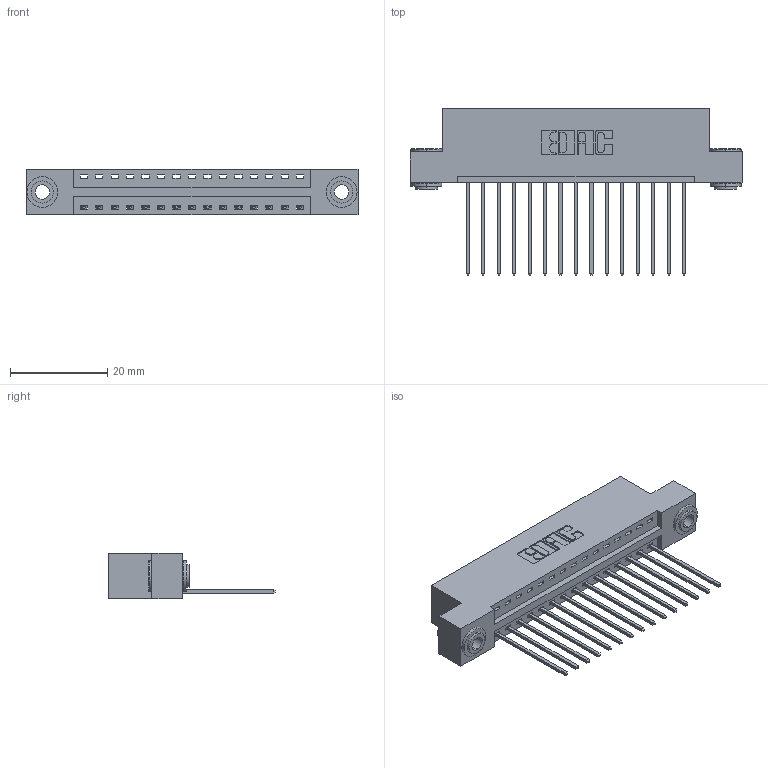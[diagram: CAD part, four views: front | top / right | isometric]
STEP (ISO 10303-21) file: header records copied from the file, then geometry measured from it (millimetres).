
FILE_DESCRIPTION (( 'STEP AP203' ), '1' );
FILE_NAME ('396-015-541-103.STEP', '2019-10-26T17:44:25', ( '' ), ( '' ), 'SwSTEP 2.0', 'SolidWorks 2016', '' );
FILE_SCHEMA (( 'CONFIG_CONTROL_DESIGN' ));
Length unit declared in the file: inch
Products named in the file (4): 345-250-002_345-250-002-102; 346 Part_Flush Mounting Lugs - 0.156 Dia-TH; 396-015-541-103; 345-292-001_345-293-141
Assembly tree (18 placements, depth 2):
  396-015-541-103
    346 Part_Flush Mounting Lugs - 0.156 Dia-TH
    345-292-001_345-293-141  x15
    345-250-002_345-250-002-102  x2
Bounding box: 68.2 x 34.29 x 9.4 mm (x, y, z)
Volume: 6411 mm3; surface area: 8236.5 mm2
Topology: 18 solids, 18 shells, 1030 faces, 3045 edges, 2006 vertices
Faces by surface type: plane 686, cylinder 336, cone 8
Entity records: 13612 total; most frequent: CARTESIAN_POINT 2320, ORIENTED_EDGE 2262, DIRECTION 2111, EDGE_CURVE 1131, LINE 915, VECTOR 915, VERTEX_POINT 750, AXIS2_PLACEMENT_3D 598
